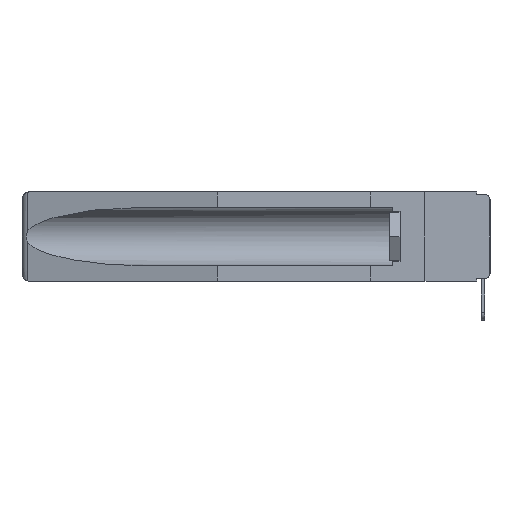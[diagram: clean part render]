
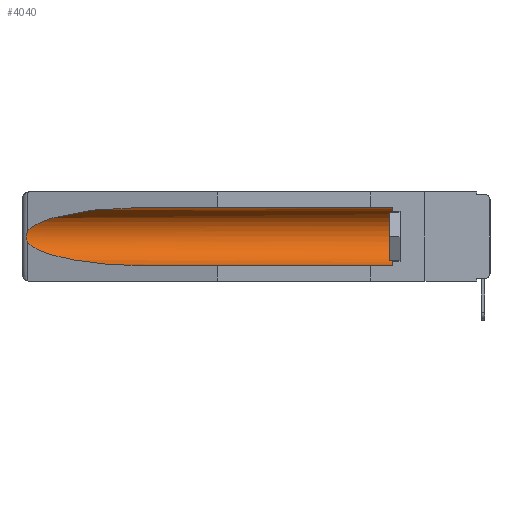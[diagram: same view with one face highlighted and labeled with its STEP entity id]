
A CAD part, left-side view. The second image highlights one B-rep face of the part: STEP entity #4040.
In plain terms, the highlighted cylindrical face has radius 2.857 mm (diameter 5.715 mm), a partial arc.
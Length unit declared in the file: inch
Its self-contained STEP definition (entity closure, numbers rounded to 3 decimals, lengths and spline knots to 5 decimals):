
#114 = CYLINDRICAL_SURFACE ( 'NONE', #18767, 0.1125 ) ;
#857 = ORIENTED_EDGE ( 'NONE', *, *, #2290, .T. ) ;
#938 = VECTOR ( 'NONE', #15673, 39.37008 ) ;
#1014 = CARTESIAN_POINT ( 'NONE',  ( 0.26597, 1.52961, -0.15275 ) ) ;
#1022 = CARTESIAN_POINT ( 'NONE',  ( 0.26537, 1.52718, -0.19328 ) ) ;
#1156 = VERTEX_POINT ( 'NONE', #11845 ) ;
#1647 = CARTESIAN_POINT ( 'NONE',  ( 0.155, -0.30754, -0.284 ) ) ;
#2290 = EDGE_CURVE ( 'NONE', #8289, #1156, #6043, .T. ) ;
#2575 = DIRECTION ( 'NONE',  ( 0., 0., 1. ) ) ;
#3169 = CARTESIAN_POINT ( 'NONE',  ( 0.155, 0.126, -0.284 ) ) ;
#3263 = CARTESIAN_POINT ( 'NONE',  ( 0.155, -0.30754, -0.1715 ) ) ;
#3294 = EDGE_CURVE ( 'NONE', #19475, #4810, #16419, .T. ) ;
#3344 = AXIS2_PLACEMENT_3D ( 'NONE', #17770, #3957, #2575 ) ;
#3399 = ORIENTED_EDGE ( 'NONE', *, *, #19124, .T. ) ;
#3530 = CARTESIAN_POINT ( 'NONE',  ( 0.155, 1.07973, -0.059 ) ) ;
#3584 = LINE ( 'NONE', #9633, #938 ) ;
#3647 = CIRCLE ( 'NONE', #3344, 0.1125 ) ;
#3957 = DIRECTION ( 'NONE',  ( 0., -1., 0. ) ) ;
#4040 = ADVANCED_FACE ( 'NONE', ( #9103 ), #114, .F. ) ;
#4133 =( BOUNDED_CURVE ( )  B_SPLINE_CURVE ( 3, ( #1022, #4265, #11608, #17680 ),
 .UNSPECIFIED., .F., .T. ) 
 B_SPLINE_CURVE_WITH_KNOTS ( ( 4, 4 ),
 ( 0.1948, 1.5708 ),
 .UNSPECIFIED. ) 
 CURVE ( )  GEOMETRIC_REPRESENTATION_ITEM ( )  RATIONAL_B_SPLINE_CURVE ( ( 1., 0.848, 0.848, 1. ) ) 
 REPRESENTATION_ITEM ( '' )  );
#4208 = CARTESIAN_POINT ( 'NONE',  ( 0.155, 1.07973, -0.284 ) ) ;
#4265 = CARTESIAN_POINT ( 'NONE',  ( 0.25451, 1.48313, -0.24835 ) ) ;
#4652 = ORIENTED_EDGE ( 'NONE', *, *, #11012, .T. ) ;
#4810 = VERTEX_POINT ( 'NONE', #4208 ) ;
#6043 = B_SPLINE_CURVE_WITH_KNOTS ( 'NONE', 3,
 ( #14270, #1014, #19173, #19283, #12984, #18872, #19068, #14368, #9807, #7138 ),
 .UNSPECIFIED., .F., .F.,
 ( 4, 2, 2, 2, 4 ),
 ( 0., 0.00029, 0.00058, 0.00087, 0.00117 ),
 .UNSPECIFIED. ) ;
#7138 = CARTESIAN_POINT ( 'NONE',  ( 0.26537, 1.52718, -0.19328 ) ) ;
#7950 = CARTESIAN_POINT ( 'NONE',  ( 0.25451, 1.48313, -0.09465 ) ) ;
#8289 = VERTEX_POINT ( 'NONE', #9658 ) ;
#8833 = EDGE_CURVE ( 'NONE', #18338, #10860, #3584, .T. ) ;
#8950 = EDGE_CURVE ( 'NONE', #19475, #18338, #3647, .T. ) ;
#9052 = EDGE_LOOP ( 'NONE', ( #3399, #857, #4652, #17808, #14348, #14618 ) ) ;
#9103 = FACE_OUTER_BOUND ( 'NONE', #9052, .T. ) ;
#9300 = DIRECTION ( 'NONE',  ( 0., 1., 0. ) ) ;
#9633 = CARTESIAN_POINT ( 'NONE',  ( 0.155, -0.30754, -0.059 ) ) ;
#9658 = CARTESIAN_POINT ( 'NONE',  ( 0.26537, 1.52718, -0.14972 ) ) ;
#9807 = CARTESIAN_POINT ( 'NONE',  ( 0.26597, 1.5296, -0.19026 ) ) ;
#10464 = DIRECTION ( 'NONE',  ( 0., 1., 0. ) ) ;
#10590 = DIRECTION ( 'NONE',  ( 0., 0., 1. ) ) ;
#10860 = VERTEX_POINT ( 'NONE', #3530 ) ;
#11012 = EDGE_CURVE ( 'NONE', #1156, #4810, #4133, .T. ) ;
#11122 = VECTOR ( 'NONE', #10464, 39.37008 ) ;
#11608 = CARTESIAN_POINT ( 'NONE',  ( 0.21114, 1.30732, -0.284 ) ) ;
#11845 = CARTESIAN_POINT ( 'NONE',  ( 0.26537, 1.52718, -0.19328 ) ) ;
#12553 = CARTESIAN_POINT ( 'NONE',  ( 0.155, 0.126, -0.059 ) ) ;
#12984 = CARTESIAN_POINT ( 'NONE',  ( 0.2675, 1.53308, -0.16763 ) ) ;
#14270 = CARTESIAN_POINT ( 'NONE',  ( 0.26537, 1.52718, -0.14972 ) ) ;
#14348 = ORIENTED_EDGE ( 'NONE', *, *, #8950, .T. ) ;
#14368 = CARTESIAN_POINT ( 'NONE',  ( 0.26655, 1.53094, -0.18657 ) ) ;
#14618 = ORIENTED_EDGE ( 'NONE', *, *, #8833, .T. ) ;
#15673 = DIRECTION ( 'NONE',  ( 0., 1., 0. ) ) ;
#16419 = LINE ( 'NONE', #1647, #11122 ) ;
#16822 =( BOUNDED_CURVE ( )  B_SPLINE_CURVE ( 3, ( #18512, #17088, #7950, #16999 ),
 .UNSPECIFIED., .F., .T. ) 
 B_SPLINE_CURVE_WITH_KNOTS ( ( 4, 4 ),
 ( 4.71239, 6.08839 ),
 .UNSPECIFIED. ) 
 CURVE ( )  GEOMETRIC_REPRESENTATION_ITEM ( )  RATIONAL_B_SPLINE_CURVE ( ( 1., 0.848, 0.848, 1. ) ) 
 REPRESENTATION_ITEM ( '' )  );
#16999 = CARTESIAN_POINT ( 'NONE',  ( 0.26537, 1.52718, -0.14972 ) ) ;
#17088 = CARTESIAN_POINT ( 'NONE',  ( 0.21114, 1.30732, -0.059 ) ) ;
#17680 = CARTESIAN_POINT ( 'NONE',  ( 0.155, 1.07973, -0.284 ) ) ;
#17770 = CARTESIAN_POINT ( 'NONE',  ( 0.155, 0.126, -0.1715 ) ) ;
#17808 = ORIENTED_EDGE ( 'NONE', *, *, #3294, .F. ) ;
#18338 = VERTEX_POINT ( 'NONE', #12553 ) ;
#18512 = CARTESIAN_POINT ( 'NONE',  ( 0.155, 1.07973, -0.059 ) ) ;
#18767 = AXIS2_PLACEMENT_3D ( 'NONE', #3263, #9300, #10590 ) ;
#18872 = CARTESIAN_POINT ( 'NONE',  ( 0.2675, 1.53308, -0.17534 ) ) ;
#19068 = CARTESIAN_POINT ( 'NONE',  ( 0.2673, 1.53269, -0.17917 ) ) ;
#19124 = EDGE_CURVE ( 'NONE', #10860, #8289, #16822, .T. ) ;
#19173 = CARTESIAN_POINT ( 'NONE',  ( 0.26654, 1.53092, -0.15636 ) ) ;
#19283 = CARTESIAN_POINT ( 'NONE',  ( 0.2673, 1.5327, -0.16383 ) ) ;
#19475 = VERTEX_POINT ( 'NONE', #3169 ) ;
